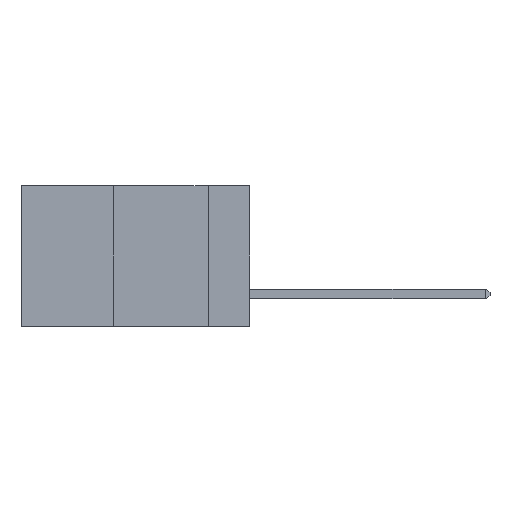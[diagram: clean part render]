
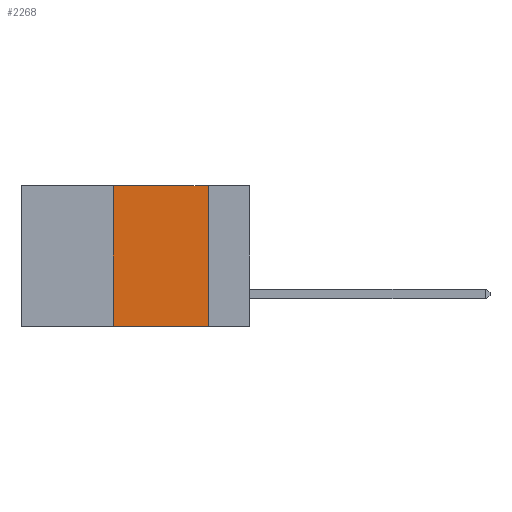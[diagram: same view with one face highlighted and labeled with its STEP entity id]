
A CAD part, left-side view. The second image highlights one B-rep face of the part: STEP entity #2268.
In plain terms, the highlighted planar face has unit normal (-1, 0, 0).
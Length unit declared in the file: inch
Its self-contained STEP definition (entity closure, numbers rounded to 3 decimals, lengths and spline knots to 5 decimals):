
#411 = CARTESIAN_POINT ( 'NONE',  ( 0., 0.36, 0. ) ) ;
#492 = VERTEX_POINT ( 'NONE', #9731 ) ;
#733 = DIRECTION ( 'NONE',  ( 0., -1., 0. ) ) ;
#839 = ORIENTED_EDGE ( 'NONE', *, *, #10342, .F. ) ;
#927 = VERTEX_POINT ( 'NONE', #8689 ) ;
#983 = ORIENTED_EDGE ( 'NONE', *, *, #5597, .F. ) ;
#1571 = CARTESIAN_POINT ( 'NONE',  ( 0., 0.6, 0. ) ) ;
#2264 = PLANE ( 'NONE',  #9653 ) ;
#2268 = ADVANCED_FACE ( 'NONE', ( #5424 ), #2264, .F. ) ;
#2601 = VECTOR ( 'NONE', #3436, 39.37008 ) ;
#2912 = LINE ( 'NONE', #411, #2601 ) ;
#3057 = DIRECTION ( 'NONE',  ( 0., -1., 0. ) ) ;
#3436 = DIRECTION ( 'NONE',  ( 0., 0., 1. ) ) ;
#3815 = VECTOR ( 'NONE', #733, 39.37008 ) ;
#4170 = EDGE_LOOP ( 'NONE', ( #6432, #983, #839, #8253 ) ) ;
#4815 = CARTESIAN_POINT ( 'NONE',  ( 0., 0.36, -0.37 ) ) ;
#5424 = FACE_OUTER_BOUND ( 'NONE', #4170, .T. ) ;
#5597 = EDGE_CURVE ( 'NONE', #492, #11470, #8990, .T. ) ;
#6432 = ORIENTED_EDGE ( 'NONE', *, *, #11055, .F. ) ;
#6651 = CARTESIAN_POINT ( 'NONE',  ( 0., 0.11, 0. ) ) ;
#6733 = LINE ( 'NONE', #10522, #11349 ) ;
#8253 = ORIENTED_EDGE ( 'NONE', *, *, #10066, .T. ) ;
#8689 = CARTESIAN_POINT ( 'NONE',  ( 0., 0.11, -0.37 ) ) ;
#8990 = LINE ( 'NONE', #9278, #3815 ) ;
#9278 = CARTESIAN_POINT ( 'NONE',  ( 0., 0.6, 0. ) ) ;
#9517 = DIRECTION ( 'NONE',  ( 1., 0., 0. ) ) ;
#9653 = AXIS2_PLACEMENT_3D ( 'NONE', #1571, #9517, #9752 ) ;
#9731 = CARTESIAN_POINT ( 'NONE',  ( 0., 0.36, 0. ) ) ;
#9752 = DIRECTION ( 'NONE',  ( 0., 0., -1. ) ) ;
#9820 = CARTESIAN_POINT ( 'NONE',  ( 0., 0.6, -0.37 ) ) ;
#10066 = EDGE_CURVE ( 'NONE', #11017, #927, #10949, .T. ) ;
#10342 = EDGE_CURVE ( 'NONE', #11017, #492, #2912, .T. ) ;
#10522 = CARTESIAN_POINT ( 'NONE',  ( 0., 0.11, 0. ) ) ;
#10668 = VECTOR ( 'NONE', #3057, 39.37008 ) ;
#10711 = DIRECTION ( 'NONE',  ( 0., 0., -1. ) ) ;
#10949 = LINE ( 'NONE', #9820, #10668 ) ;
#11017 = VERTEX_POINT ( 'NONE', #4815 ) ;
#11055 = EDGE_CURVE ( 'NONE', #11470, #927, #6733, .T. ) ;
#11349 = VECTOR ( 'NONE', #10711, 39.37008 ) ;
#11470 = VERTEX_POINT ( 'NONE', #6651 ) ;
